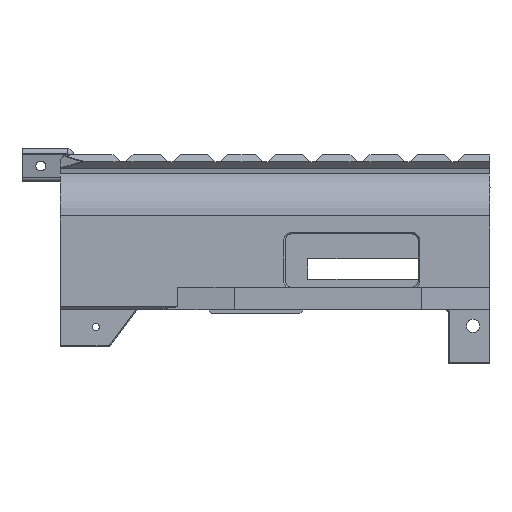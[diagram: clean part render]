
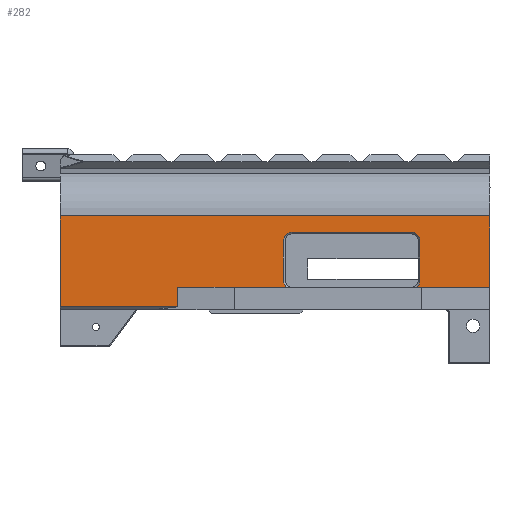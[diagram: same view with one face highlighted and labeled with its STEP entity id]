
A CAD part, top view. The second image highlights one B-rep face of the part: STEP entity #282.
In plain terms, the highlighted planar face has unit normal (0, 0, 1).
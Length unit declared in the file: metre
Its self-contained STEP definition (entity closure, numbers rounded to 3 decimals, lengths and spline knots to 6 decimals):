
#282=ADVANCED_FACE('11:2741',(#791),#792,.T.);
#791=FACE_OUTER_BOUND('',#1473,.T.);
#792=PLANE('',#1474);
#1473=EDGE_LOOP('',(#3342,#3343,#3344,#3345,#3346,#3347,#3348,#3349,#3350,#3351,#3352,#3353,#3354,#3355));
#1474=AXIS2_PLACEMENT_3D('',#3356,#3357,#3358);
#3342=ORIENTED_EDGE('',*,*,#4341,.F.);
#3343=ORIENTED_EDGE('',*,*,#4344,.F.);
#3344=ORIENTED_EDGE('',*,*,#4345,.F.);
#3345=ORIENTED_EDGE('',*,*,#4302,.T.);
#3346=ORIENTED_EDGE('',*,*,#4319,.T.);
#3347=ORIENTED_EDGE('',*,*,#4323,.T.);
#3348=ORIENTED_EDGE('',*,*,#4342,.F.);
#3349=ORIENTED_EDGE('',*,*,#4116,.T.);
#3350=ORIENTED_EDGE('',*,*,#4115,.T.);
#3351=ORIENTED_EDGE('',*,*,#4112,.T.);
#3352=ORIENTED_EDGE('',*,*,#4111,.T.);
#3353=ORIENTED_EDGE('',*,*,#4108,.T.);
#3354=ORIENTED_EDGE('',*,*,#4107,.T.);
#3355=ORIENTED_EDGE('',*,*,#4103,.T.);
#3356=CARTESIAN_POINT('',(-0.020072,0.047361,0.0211));
#3357=DIRECTION('',(0.,0.,1.0));
#3358=DIRECTION('',(1.0,0.0,0.));
#4103=EDGE_CURVE('11:3848',#5113,#5114,#5115,.T.);
#4107=EDGE_CURVE('11:3845',#5118,#5113,#5120,.T.);
#4108=EDGE_CURVE('11:3839',#5121,#5118,#5122,.T.);
#4111=EDGE_CURVE('11:3833',#5124,#5121,#5126,.T.);
#4112=EDGE_CURVE('11:3827',#5127,#5124,#5128,.T.);
#4115=EDGE_CURVE('11:3821',#5130,#5127,#5132,.T.);
#4116=EDGE_CURVE('11:3812',#5133,#5130,#5134,.T.);
#4302=EDGE_CURVE('11:4436',#5406,#5404,#5407,.T.);
#4319=EDGE_CURVE('11:4439',#5404,#5435,#5438,.T.);
#4323=EDGE_CURVE('11:4442',#5435,#5441,#5443,.T.);
#4341=EDGE_CURVE('11:4382',#5466,#5114,#5467,.T.);
#4342=EDGE_CURVE('11:4385',#5133,#5441,#5468,.T.);
#4344=EDGE_CURVE('11:3047',#5470,#5466,#5471,.T.);
#4345=EDGE_CURVE('11:4433',#5406,#5470,#5472,.T.);
#5113=VERTEX_POINT('',#6644);
#5114=VERTEX_POINT('',#6645);
#5115=CIRCLE('',#6646,0.0038);
#5118=VERTEX_POINT('',#6660);
#5120=LINE('',#6663,#6664);
#5121=VERTEX_POINT('',#6665);
#5122=CIRCLE('',#6666,0.0038);
#5124=VERTEX_POINT('',#6669);
#5126=LINE('',#6672,#6673);
#5127=VERTEX_POINT('',#6674);
#5128=CIRCLE('',#6675,0.0038);
#5130=VERTEX_POINT('',#6678);
#5132=LINE('',#6681,#6682);
#5133=VERTEX_POINT('',#6683);
#5134=CIRCLE('',#6684,0.0038);
#5404=VERTEX_POINT('',#7196);
#5406=VERTEX_POINT('',#7199);
#5407=LINE('',#7200,#7201);
#5435=VERTEX_POINT('',#7238);
#5438=LINE('',#7242,#7243);
#5441=VERTEX_POINT('',#7248);
#5443=LINE('',#7251,#7252);
#5466=VERTEX_POINT('',#7285);
#5467=LINE('',#7286,#7287);
#5468=LINE('',#7288,#7289);
#5470=VERTEX_POINT('',#7292);
#5471=LINE('',#7293,#7294);
#5472=LINE('',#7295,#7296);
#6644=CARTESIAN_POINT('',(-0.019378,0.018811,0.0211));
#6645=CARTESIAN_POINT('',(-0.020846,0.015811,0.0211));
#6646=AXIS2_PLACEMENT_3D('',#8003,#8004,#8005);
#6660=CARTESIAN_POINT('',(-0.019378,0.036397,0.0211));
#6663=CARTESIAN_POINT('',(-0.019378,0.047361,0.0211));
#6664=VECTOR('',#8008,1.0);
#6665=CARTESIAN_POINT('',(-0.023178,0.040197,0.0211));
#6666=AXIS2_PLACEMENT_3D('',#8009,#8010,#8011);
#6669=CARTESIAN_POINT('',(-0.076022,0.040197,0.0211));
#6672=CARTESIAN_POINT('',(-0.020072,0.040197,0.0211));
#6673=VECTOR('',#8014,1.0);
#6674=CARTESIAN_POINT('',(-0.079822,0.036397,0.0211));
#6675=AXIS2_PLACEMENT_3D('',#8015,#8016,#8017);
#6678=CARTESIAN_POINT('',(-0.079822,0.018811,0.0211));
#6681=CARTESIAN_POINT('',(-0.079822,0.047361,0.0211));
#6682=VECTOR('',#8020,1.0);
#6683=CARTESIAN_POINT('',(-0.078355,0.015811,0.0211));
#6684=AXIS2_PLACEMENT_3D('',#8021,#8022,#8023);
#7196=CARTESIAN_POINT('',(-0.178704,0.007104,0.0211));
#7199=CARTESIAN_POINT('',(-0.178704,0.047361,0.0211));
#7200=CARTESIAN_POINT('',(-0.178704,0.030072,0.0211));
#7201=VECTOR('',#8206,1.0);
#7238=CARTESIAN_POINT('',(-0.126814,0.007104,0.0211));
#7242=CARTESIAN_POINT('',(-0.089922,0.007104,0.0211));
#7243=VECTOR('',#8235,1.0);
#7248=CARTESIAN_POINT('',(-0.126814,0.015811,0.0211));
#7251=CARTESIAN_POINT('',(-0.126814,0.047361,0.0211));
#7252=VECTOR('',#8239,1.0);
#7285=CARTESIAN_POINT('',(0.011678,0.015811,0.0211));
#7286=CARTESIAN_POINT('',(-0.106587,0.015811,0.0211));
#7287=VECTOR('',#8271,1.0);
#7288=CARTESIAN_POINT('',(-0.106587,0.015811,0.0211));
#7289=VECTOR('',#8272,1.0);
#7292=CARTESIAN_POINT('',(0.011678,0.047361,0.0211));
#7293=CARTESIAN_POINT('',(0.011678,0.047361,0.0211));
#7294=VECTOR('',#8274,1.0);
#7295=CARTESIAN_POINT('',(-0.020072,0.047361,0.0211));
#7296=VECTOR('',#8275,1.0);
#8003=CARTESIAN_POINT('',(-0.023178,0.018811,0.0211));
#8004=DIRECTION('',(0.,0.,-1.0));
#8005=DIRECTION('',(1.0,0.,0.));
#8008=DIRECTION('',(0.,-1.0,0.));
#8009=CARTESIAN_POINT('',(-0.023178,0.036397,0.0211));
#8010=DIRECTION('',(0.,0.,-1.0));
#8011=DIRECTION('',(1.0,0.,0.));
#8014=DIRECTION('',(1.0,0.0,0.));
#8015=CARTESIAN_POINT('',(-0.076022,0.036397,0.0211));
#8016=DIRECTION('',(0.,0.,-1.0));
#8017=DIRECTION('',(1.0,0.,0.));
#8020=DIRECTION('',(0.,1.0,0.));
#8021=CARTESIAN_POINT('',(-0.076022,0.018811,0.0211));
#8022=DIRECTION('',(0.,0.,-1.0));
#8023=DIRECTION('',(1.0,0.,0.));
#8206=DIRECTION('',(0.0,-1.0,-0.0));
#8235=DIRECTION('',(1.0,0.,0.));
#8239=DIRECTION('',(0.,1.0,0.));
#8271=DIRECTION('',(-1.0,0.,0.));
#8272=DIRECTION('',(-1.0,0.,0.));
#8274=DIRECTION('',(0.,-1.0,0.));
#8275=DIRECTION('',(1.0,0.0,0.));
